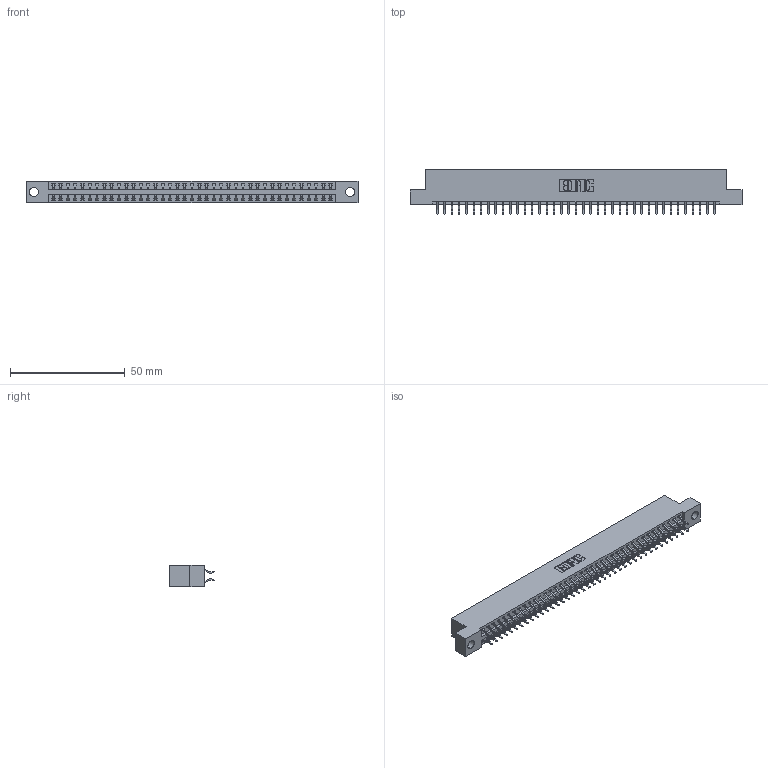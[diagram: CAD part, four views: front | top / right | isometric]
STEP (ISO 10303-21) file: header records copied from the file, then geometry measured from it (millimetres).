
FILE_DESCRIPTION (( 'STEP AP203' ), '1' );
FILE_NAME ('346-078-556-204.STEP', '2022-05-25T14:29:51', ( '' ), ( '' ), 'SwSTEP 2.0', 'SolidWorks 2020', '' );
FILE_SCHEMA (( 'CONFIG_CONTROL_DESIGN' ));
Length unit declared in the file: inch
Products named in the file (3): 346-078-556-204; 346 Part_Flush Mounting Lugs - 0.156 Dia-TH; 345-292-001_556 Tail
Assembly tree (79 placements, depth 2):
  346-078-556-204
    346 Part_Flush Mounting Lugs - 0.156 Dia-TH
    345-292-001_556 Tail  x78
Bounding box: 144.4 x 19.57 x 9.4 mm (x, y, z)
Volume: 13948.4 mm3; surface area: 18901.2 mm2
Topology: 79 solids, 79 shells, 4660 faces, 13859 edges, 9134 vertices
Faces by surface type: plane 3132, cylinder 1528
Entity records: 26495 total; most frequent: CARTESIAN_POINT 4390, ORIENTED_EDGE 4310, DIRECTION 3907, EDGE_CURVE 2155, VECTOR 1859, LINE 1859, VERTEX_POINT 1434, AXIS2_PLACEMENT_3D 1024
